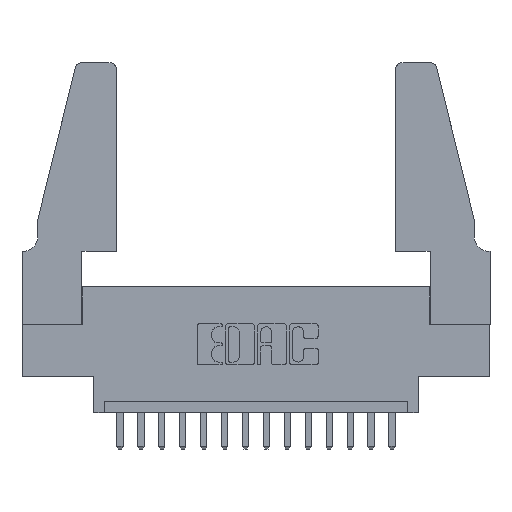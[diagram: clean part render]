
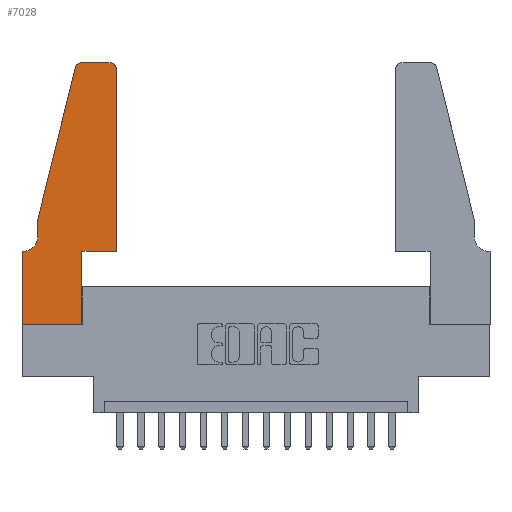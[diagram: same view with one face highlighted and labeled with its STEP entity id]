
A CAD part, top view. The second image highlights one B-rep face of the part: STEP entity #7028.
In plain terms, the highlighted planar face has unit normal (0, 0, 1).
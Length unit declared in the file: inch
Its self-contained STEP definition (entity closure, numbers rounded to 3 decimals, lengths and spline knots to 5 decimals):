
#406 = CARTESIAN_POINT ( 'NONE',  ( 0.2865, 0.35, 0.37 ) ) ;
#525 = CIRCLE ( 'NONE', #6024, 0.03 ) ;
#721 = EDGE_CURVE ( 'NONE', #13134, #3421, #8308, .T. ) ;
#778 = ORIENTED_EDGE ( 'NONE', *, *, #13313, .T. ) ;
#894 = EDGE_CURVE ( 'NONE', #10882, #6172, #2228, .T. ) ;
#936 = EDGE_CURVE ( 'NONE', #15903, #10882, #6913, .T. ) ;
#940 = DIRECTION ( 'NONE',  ( -1., 0., 0. ) ) ;
#997 = ORIENTED_EDGE ( 'NONE', *, *, #12267, .T. ) ;
#1698 = LINE ( 'NONE', #2068, #7148 ) ;
#1746 = LINE ( 'NONE', #10931, #13459 ) ;
#2030 = ORIENTED_EDGE ( 'NONE', *, *, #894, .T. ) ;
#2068 = CARTESIAN_POINT ( 'NONE',  ( 0.0755, 0.5, 0.37 ) ) ;
#2086 = VERTEX_POINT ( 'NONE', #7925 ) ;
#2088 = CARTESIAN_POINT ( 'NONE',  ( 0.4205, 1.25, 0.37 ) ) ;
#2153 = EDGE_CURVE ( 'NONE', #3161, #15903, #14134, .T. ) ;
#2213 = CARTESIAN_POINT ( 'NONE',  ( 0.0055, 0.35, 0.37 ) ) ;
#2228 = LINE ( 'NONE', #5746, #12920 ) ;
#2345 = CARTESIAN_POINT ( 'NONE',  ( 0., 0.35, 0.37 ) ) ;
#2570 = VECTOR ( 'NONE', #2729, 39.37008 ) ;
#2729 = DIRECTION ( 'NONE',  ( 0., -1., 0. ) ) ;
#2920 = VERTEX_POINT ( 'NONE', #14193 ) ;
#2986 = DIRECTION ( 'NONE',  ( 0., 0., 1. ) ) ;
#3023 = VECTOR ( 'NONE', #11749, 39.37008 ) ;
#3161 = VERTEX_POINT ( 'NONE', #12296 ) ;
#3408 = DIRECTION ( 'NONE',  ( 0., 0., 1. ) ) ;
#3421 = VERTEX_POINT ( 'NONE', #2213 ) ;
#3690 = EDGE_CURVE ( 'NONE', #12288, #9628, #525, .T. ) ;
#3777 = LINE ( 'NONE', #8820, #6791 ) ;
#4109 = FACE_OUTER_BOUND ( 'NONE', #5028, .T. ) ;
#4139 = CARTESIAN_POINT ( 'NONE',  ( 0.284, 1.22, 0.37 ) ) ;
#4779 = EDGE_CURVE ( 'NONE', #9628, #11335, #8989, .T. ) ;
#4959 = LINE ( 'NONE', #8550, #12817 ) ;
#5028 = EDGE_LOOP ( 'NONE', ( #16114, #997, #8300, #7253, #16251, #8776, #5233, #14271, #2030, #12021, #778, #8413 ) ) ;
#5106 = AXIS2_PLACEMENT_3D ( 'NONE', #2345, #8832, #15298 ) ;
#5233 = ORIENTED_EDGE ( 'NONE', *, *, #2153, .T. ) ;
#5327 = EDGE_CURVE ( 'NONE', #3421, #3161, #3777, .T. ) ;
#5746 = CARTESIAN_POINT ( 'NONE',  ( 0.2865, 0.35, 0.37 ) ) ;
#5844 = DIRECTION ( 'NONE',  ( 1., 0., 0. ) ) ;
#6024 = AXIS2_PLACEMENT_3D ( 'NONE', #14679, #3408, #16256 ) ;
#6172 = VERTEX_POINT ( 'NONE', #406 ) ;
#6402 = CARTESIAN_POINT ( 'NONE',  ( 0., 0., 0.37 ) ) ;
#6412 = EDGE_CURVE ( 'NONE', #2086, #2920, #1698, .T. ) ;
#6551 = CARTESIAN_POINT ( 'NONE',  ( 0.0755, 0.5, 0.37 ) ) ;
#6791 = VECTOR ( 'NONE', #940, 39.37008 ) ;
#6913 = LINE ( 'NONE', #10645, #7879 ) ;
#6980 = VECTOR ( 'NONE', #15779, 39.37008 ) ;
#7028 = ADVANCED_FACE ( 'NONE', ( #4109 ), #15197, .T. ) ;
#7148 = VECTOR ( 'NONE', #9844, 39.37008 ) ;
#7253 = ORIENTED_EDGE ( 'NONE', *, *, #12088, .T. ) ;
#7482 = CARTESIAN_POINT ( 'NONE',  ( 0.284, 1.25, 0.37 ) ) ;
#7879 = VECTOR ( 'NONE', #15692, 39.37008 ) ;
#7925 = CARTESIAN_POINT ( 'NONE',  ( 0.25487, 1.22718, 0.37 ) ) ;
#8112 = DIRECTION ( 'NONE',  ( 0., 1., 0. ) ) ;
#8300 = ORIENTED_EDGE ( 'NONE', *, *, #6412, .T. ) ;
#8308 = CIRCLE ( 'NONE', #11291, 0.07 ) ;
#8413 = ORIENTED_EDGE ( 'NONE', *, *, #3690, .T. ) ;
#8550 = CARTESIAN_POINT ( 'NONE',  ( 0.4505, 0.35, 0.37 ) ) ;
#8776 = ORIENTED_EDGE ( 'NONE', *, *, #5327, .T. ) ;
#8820 = CARTESIAN_POINT ( 'NONE',  ( 0.0755, 0.35, 0.37 ) ) ;
#8832 = DIRECTION ( 'NONE',  ( 0., 0., 1. ) ) ;
#8989 = LINE ( 'NONE', #16729, #6980 ) ;
#9116 = CARTESIAN_POINT ( 'NONE',  ( 0.4505, 0.35, 0.37 ) ) ;
#9628 = VERTEX_POINT ( 'NONE', #2088 ) ;
#9844 = DIRECTION ( 'NONE',  ( -0.239, -0.971, 0. ) ) ;
#10179 = DIRECTION ( 'NONE',  ( 0., 1., 0. ) ) ;
#10645 = CARTESIAN_POINT ( 'NONE',  ( 0., 0., 0.37 ) ) ;
#10882 = VERTEX_POINT ( 'NONE', #15706 ) ;
#10931 = CARTESIAN_POINT ( 'NONE',  ( 0.4505, 0.35, 0.37 ) ) ;
#11024 = CIRCLE ( 'NONE', #16135, 0.03 ) ;
#11039 = CARTESIAN_POINT ( 'NONE',  ( 0.0755, 0.42, 0.37 ) ) ;
#11155 = EDGE_CURVE ( 'NONE', #6172, #13565, #1746, .T. ) ;
#11291 = AXIS2_PLACEMENT_3D ( 'NONE', #14178, #12873, #12661 ) ;
#11335 = VERTEX_POINT ( 'NONE', #7482 ) ;
#11749 = DIRECTION ( 'NONE',  ( 0., -1., 0. ) ) ;
#12021 = ORIENTED_EDGE ( 'NONE', *, *, #11155, .T. ) ;
#12023 = LINE ( 'NONE', #6551, #2570 ) ;
#12088 = EDGE_CURVE ( 'NONE', #2920, #13134, #12023, .T. ) ;
#12267 = EDGE_CURVE ( 'NONE', #11335, #2086, #11024, .T. ) ;
#12288 = VERTEX_POINT ( 'NONE', #14491 ) ;
#12296 = CARTESIAN_POINT ( 'NONE',  ( 0., 0.35, 0.37 ) ) ;
#12661 = DIRECTION ( 'NONE',  ( -1., 0., 0. ) ) ;
#12817 = VECTOR ( 'NONE', #10179, 39.37008 ) ;
#12873 = DIRECTION ( 'NONE',  ( 0., 0., -1. ) ) ;
#12920 = VECTOR ( 'NONE', #8112, 39.37008 ) ;
#13134 = VERTEX_POINT ( 'NONE', #11039 ) ;
#13313 = EDGE_CURVE ( 'NONE', #13565, #12288, #4959, .T. ) ;
#13459 = VECTOR ( 'NONE', #5844, 39.37008 ) ;
#13565 = VERTEX_POINT ( 'NONE', #9116 ) ;
#14134 = LINE ( 'NONE', #6402, #3023 ) ;
#14178 = CARTESIAN_POINT ( 'NONE',  ( 0.0055, 0.42, 0.37 ) ) ;
#14193 = CARTESIAN_POINT ( 'NONE',  ( 0.0755, 0.5, 0.37 ) ) ;
#14234 = CARTESIAN_POINT ( 'NONE',  ( 0., 0., 0.37 ) ) ;
#14271 = ORIENTED_EDGE ( 'NONE', *, *, #936, .T. ) ;
#14442 = DIRECTION ( 'NONE',  ( 1., 0., 0. ) ) ;
#14491 = CARTESIAN_POINT ( 'NONE',  ( 0.4505, 1.22, 0.37 ) ) ;
#14679 = CARTESIAN_POINT ( 'NONE',  ( 0.4205, 1.22, 0.37 ) ) ;
#15197 = PLANE ( 'NONE',  #5106 ) ;
#15298 = DIRECTION ( 'NONE',  ( 1., 0., 0. ) ) ;
#15692 = DIRECTION ( 'NONE',  ( 1., 0., 0. ) ) ;
#15706 = CARTESIAN_POINT ( 'NONE',  ( 0.2865, 0., 0.37 ) ) ;
#15779 = DIRECTION ( 'NONE',  ( -1., 0., 0. ) ) ;
#15903 = VERTEX_POINT ( 'NONE', #14234 ) ;
#16114 = ORIENTED_EDGE ( 'NONE', *, *, #4779, .T. ) ;
#16135 = AXIS2_PLACEMENT_3D ( 'NONE', #4139, #2986, #14442 ) ;
#16251 = ORIENTED_EDGE ( 'NONE', *, *, #721, .T. ) ;
#16256 = DIRECTION ( 'NONE',  ( 1., 0., 0. ) ) ;
#16729 = CARTESIAN_POINT ( 'NONE',  ( 0.2605, 1.25, 0.37 ) ) ;
